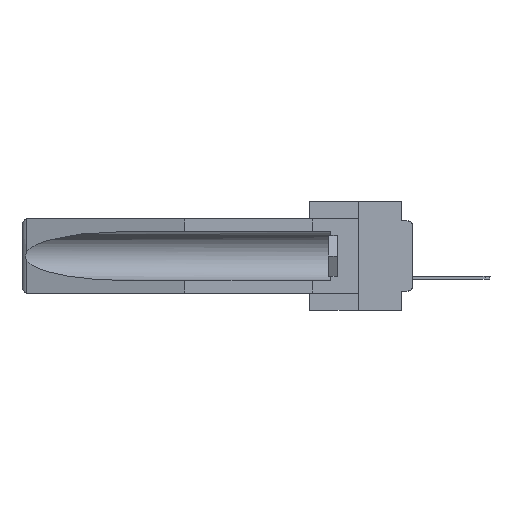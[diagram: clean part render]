
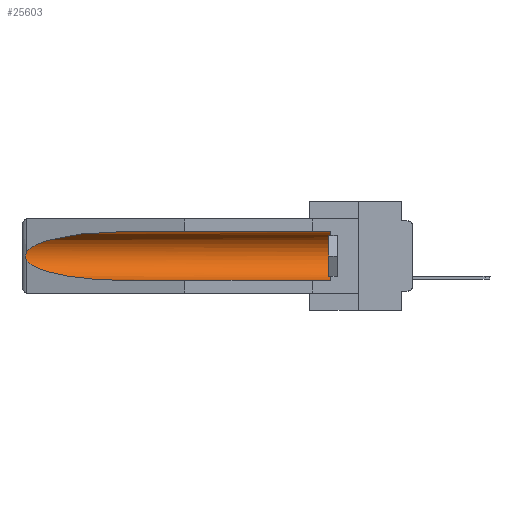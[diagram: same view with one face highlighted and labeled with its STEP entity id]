
A CAD part, left-side view. The second image highlights one B-rep face of the part: STEP entity #25603.
In plain terms, the highlighted cylindrical face has radius 2.857 mm (diameter 5.715 mm), a partial arc.
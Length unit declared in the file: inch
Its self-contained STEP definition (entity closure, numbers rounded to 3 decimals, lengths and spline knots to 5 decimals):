
#1167 = CARTESIAN_POINT ( 'NONE',  ( 0.25451, 1.48313, -0.24835 ) ) ;
#1523 = FACE_OUTER_BOUND ( 'NONE', #4997, .T. ) ;
#1603 = LINE ( 'NONE', #22158, #14723 ) ;
#2036 = ORIENTED_EDGE ( 'NONE', *, *, #24099, .T. ) ;
#2193 = CARTESIAN_POINT ( 'NONE',  ( 0.155, 1.07973, -0.059 ) ) ;
#3725 = CARTESIAN_POINT ( 'NONE',  ( 0.2675, 1.53308, -0.17534 ) ) ;
#4201 = CARTESIAN_POINT ( 'NONE',  ( 0.21114, 1.30732, -0.284 ) ) ;
#4519 = CARTESIAN_POINT ( 'NONE',  ( 0.26537, 1.52718, -0.14972 ) ) ;
#4997 = EDGE_LOOP ( 'NONE', ( #11931, #33027, #2036, #13963, #9437, #22268 ) ) ;
#5124 = CARTESIAN_POINT ( 'NONE',  ( 0.155, 0.126, -0.1715 ) ) ;
#5532 = VERTEX_POINT ( 'NONE', #20525 ) ;
#5723 =( BOUNDED_CURVE ( )  B_SPLINE_CURVE ( 3, ( #14820, #1167, #4201, #27113 ),
 .UNSPECIFIED., .F., .T. ) 
 B_SPLINE_CURVE_WITH_KNOTS ( ( 4, 4 ),
 ( 0.1948, 1.5708 ),
 .UNSPECIFIED. ) 
 CURVE ( )  GEOMETRIC_REPRESENTATION_ITEM ( )  RATIONAL_B_SPLINE_CURVE ( ( 1., 0.848, 0.848, 1. ) ) 
 REPRESENTATION_ITEM ( '' )  );
#5752 = CARTESIAN_POINT ( 'NONE',  ( 0.26655, 1.53094, -0.18657 ) ) ;
#5757 = CARTESIAN_POINT ( 'NONE',  ( 0.26537, 1.52718, -0.19328 ) ) ;
#6082 = CARTESIAN_POINT ( 'NONE',  ( 0.26597, 1.52961, -0.15275 ) ) ;
#6322 = B_SPLINE_CURVE_WITH_KNOTS ( 'NONE', 3,
 ( #21270, #6082, #26981, #19083, #29508, #3725, #8605, #5752, #29330, #14004 ),
 .UNSPECIFIED., .F., .F.,
 ( 4, 2, 2, 2, 4 ),
 ( 0., 0.00029, 0.00058, 0.00087, 0.00117 ),
 .UNSPECIFIED. ) ;
#7046 = CARTESIAN_POINT ( 'NONE',  ( 0.21114, 1.30732, -0.059 ) ) ;
#7818 = DIRECTION ( 'NONE',  ( 0., 0., 1. ) ) ;
#8001 = EDGE_CURVE ( 'NONE', #10552, #22889, #20820, .T. ) ;
#8605 = CARTESIAN_POINT ( 'NONE',  ( 0.2673, 1.53269, -0.17917 ) ) ;
#8989 = DIRECTION ( 'NONE',  ( 0., 1., 0. ) ) ;
#9229 = AXIS2_PLACEMENT_3D ( 'NONE', #11787, #9418, #29982 ) ;
#9418 = DIRECTION ( 'NONE',  ( 0., 1., 0. ) ) ;
#9437 = ORIENTED_EDGE ( 'NONE', *, *, #8001, .T. ) ;
#9703 = VERTEX_POINT ( 'NONE', #5757 ) ;
#10390 = VERTEX_POINT ( 'NONE', #2193 ) ;
#10552 = VERTEX_POINT ( 'NONE', #31630 ) ;
#10568 = AXIS2_PLACEMENT_3D ( 'NONE', #5124, #13364, #7818 ) ;
#11690 = EDGE_CURVE ( 'NONE', #22889, #10390, #23405, .T. ) ;
#11787 = CARTESIAN_POINT ( 'NONE',  ( 0.155, -0.30754, -0.1715 ) ) ;
#11931 = ORIENTED_EDGE ( 'NONE', *, *, #32319, .T. ) ;
#13364 = DIRECTION ( 'NONE',  ( 0., -1., 0. ) ) ;
#13703 =( BOUNDED_CURVE ( )  B_SPLINE_CURVE ( 3, ( #30140, #7046, #27606, #4519 ),
 .UNSPECIFIED., .F., .F. ) 
 B_SPLINE_CURVE_WITH_KNOTS ( ( 4, 4 ),
 ( 4.71239, 6.08839 ),
 .UNSPECIFIED. ) 
 CURVE ( )  GEOMETRIC_REPRESENTATION_ITEM ( )  RATIONAL_B_SPLINE_CURVE ( ( 1., 0.848, 0.848, 1. ) ) 
 REPRESENTATION_ITEM ( '' )  );
#13963 = ORIENTED_EDGE ( 'NONE', *, *, #16644, .F. ) ;
#14004 = CARTESIAN_POINT ( 'NONE',  ( 0.26537, 1.52718, -0.19328 ) ) ;
#14386 = CARTESIAN_POINT ( 'NONE',  ( 0.155, 1.07973, -0.284 ) ) ;
#14723 = VECTOR ( 'NONE', #8989, 39.37008 ) ;
#14820 = CARTESIAN_POINT ( 'NONE',  ( 0.26537, 1.52718, -0.19328 ) ) ;
#15438 = VERTEX_POINT ( 'NONE', #14386 ) ;
#16644 = EDGE_CURVE ( 'NONE', #10552, #15438, #1603, .T. ) ;
#18508 = DIRECTION ( 'NONE',  ( 0., 1., 0. ) ) ;
#19083 = CARTESIAN_POINT ( 'NONE',  ( 0.2673, 1.5327, -0.16383 ) ) ;
#20525 = CARTESIAN_POINT ( 'NONE',  ( 0.26537, 1.52718, -0.14972 ) ) ;
#20820 = CIRCLE ( 'NONE', #10568, 0.1125 ) ;
#20889 = CARTESIAN_POINT ( 'NONE',  ( 0.155, -0.30754, -0.059 ) ) ;
#21270 = CARTESIAN_POINT ( 'NONE',  ( 0.26537, 1.52718, -0.14972 ) ) ;
#21474 = VECTOR ( 'NONE', #18508, 39.37008 ) ;
#22158 = CARTESIAN_POINT ( 'NONE',  ( 0.155, -0.30754, -0.284 ) ) ;
#22268 = ORIENTED_EDGE ( 'NONE', *, *, #11690, .T. ) ;
#22889 = VERTEX_POINT ( 'NONE', #27241 ) ;
#23405 = LINE ( 'NONE', #20889, #21474 ) ;
#24099 = EDGE_CURVE ( 'NONE', #9703, #15438, #5723, .T. ) ;
#25603 = ADVANCED_FACE ( 'NONE', ( #1523 ), #30157, .F. ) ;
#25790 = EDGE_CURVE ( 'NONE', #5532, #9703, #6322, .T. ) ;
#26981 = CARTESIAN_POINT ( 'NONE',  ( 0.26654, 1.53092, -0.15636 ) ) ;
#27113 = CARTESIAN_POINT ( 'NONE',  ( 0.155, 1.07973, -0.284 ) ) ;
#27241 = CARTESIAN_POINT ( 'NONE',  ( 0.155, 0.126, -0.059 ) ) ;
#27606 = CARTESIAN_POINT ( 'NONE',  ( 0.25451, 1.48313, -0.09465 ) ) ;
#29330 = CARTESIAN_POINT ( 'NONE',  ( 0.26597, 1.5296, -0.19026 ) ) ;
#29508 = CARTESIAN_POINT ( 'NONE',  ( 0.2675, 1.53308, -0.16763 ) ) ;
#29982 = DIRECTION ( 'NONE',  ( 0., 0., 1. ) ) ;
#30140 = CARTESIAN_POINT ( 'NONE',  ( 0.155, 1.07973, -0.059 ) ) ;
#30157 = CYLINDRICAL_SURFACE ( 'NONE', #9229, 0.1125 ) ;
#31630 = CARTESIAN_POINT ( 'NONE',  ( 0.155, 0.126, -0.284 ) ) ;
#32319 = EDGE_CURVE ( 'NONE', #10390, #5532, #13703, .T. ) ;
#33027 = ORIENTED_EDGE ( 'NONE', *, *, #25790, .T. ) ;
